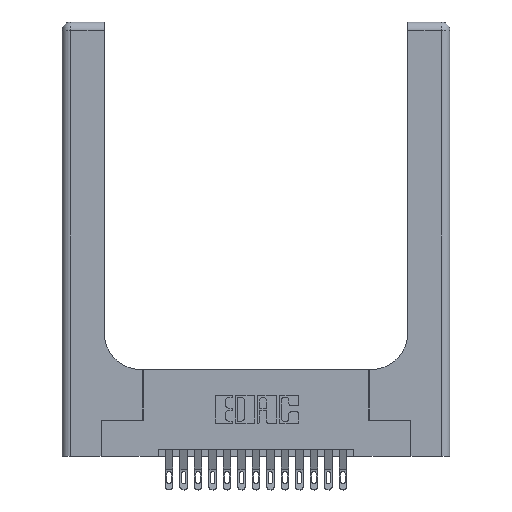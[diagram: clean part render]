
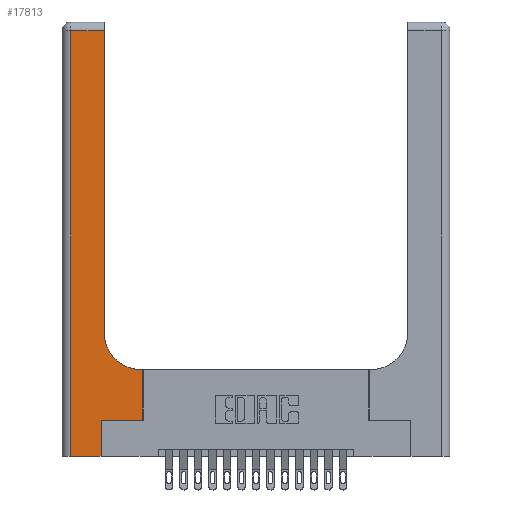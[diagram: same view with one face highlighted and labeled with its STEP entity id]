
A CAD part, top view. The second image highlights one B-rep face of the part: STEP entity #17813.
In plain terms, the highlighted planar face has unit normal (0, 0, 1).
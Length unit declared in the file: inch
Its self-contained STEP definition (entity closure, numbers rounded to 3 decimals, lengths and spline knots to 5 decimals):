
#219 = VERTEX_POINT ( 'NONE', #9522 ) ;
#544 = VERTEX_POINT ( 'NONE', #1784 ) ;
#628 = AXIS2_PLACEMENT_3D ( 'NONE', #1355, #11418, #13408 ) ;
#735 = LINE ( 'NONE', #16271, #17061 ) ;
#807 = DIRECTION ( 'NONE',  ( 1., 0., 0. ) ) ;
#1086 = EDGE_LOOP ( 'NONE', ( #16176, #7851, #3524, #15722, #14013, #7031, #16193, #15386, #12107 ) ) ;
#1355 = CARTESIAN_POINT ( 'NONE',  ( 0., 3., 0.37 ) ) ;
#1466 = LINE ( 'NONE', #12705, #5020 ) ;
#1563 = CARTESIAN_POINT ( 'NONE',  ( 0.06, 2.94, 0.37 ) ) ;
#1784 = CARTESIAN_POINT ( 'NONE',  ( 0.2915, 0.85, 0.37 ) ) ;
#1847 = EDGE_CURVE ( 'NONE', #13641, #544, #18975, .T. ) ;
#1978 = CARTESIAN_POINT ( 'NONE',  ( 0.5585, 0.6, 0.37 ) ) ;
#2128 = CARTESIAN_POINT ( 'NONE',  ( 0.5415, 0.6, 0.37 ) ) ;
#2140 = CARTESIAN_POINT ( 'NONE',  ( 0.269, 0.25, 0.37 ) ) ;
#2630 = VECTOR ( 'NONE', #8800, 39.37008 ) ;
#3524 = ORIENTED_EDGE ( 'NONE', *, *, #8120, .T. ) ;
#3537 = VECTOR ( 'NONE', #17474, 39.37008 ) ;
#4031 = LINE ( 'NONE', #13912, #3537 ) ;
#5020 = VECTOR ( 'NONE', #807, 39.37008 ) ;
#5067 = CARTESIAN_POINT ( 'NONE',  ( 0.2915, 0.6, 0.37 ) ) ;
#5186 = CARTESIAN_POINT ( 'NONE',  ( 0.06, 3., 0.37 ) ) ;
#5453 = AXIS2_PLACEMENT_3D ( 'NONE', #8823, #17914, #10262 ) ;
#6073 = VECTOR ( 'NONE', #14108, 39.37008 ) ;
#7031 = ORIENTED_EDGE ( 'NONE', *, *, #15122, .T. ) ;
#7089 = CARTESIAN_POINT ( 'NONE',  ( 0.269, 0., 0.37 ) ) ;
#7225 = DIRECTION ( 'NONE',  ( 0., 1., 0. ) ) ;
#7851 = ORIENTED_EDGE ( 'NONE', *, *, #9613, .T. ) ;
#8120 = EDGE_CURVE ( 'NONE', #12948, #219, #14992, .T. ) ;
#8372 = LINE ( 'NONE', #5067, #12856 ) ;
#8697 = EDGE_CURVE ( 'NONE', #14667, #13161, #735, .T. ) ;
#8800 = DIRECTION ( 'NONE',  ( -1., 0., 0. ) ) ;
#8823 = CARTESIAN_POINT ( 'NONE',  ( 0.5415, 0.85, 0.37 ) ) ;
#8880 = FACE_OUTER_BOUND ( 'NONE', #1086, .T. ) ;
#8973 = VERTEX_POINT ( 'NONE', #1978 ) ;
#9394 = LINE ( 'NONE', #2140, #6073 ) ;
#9522 = CARTESIAN_POINT ( 'NONE',  ( 0.06, 0., 0.37 ) ) ;
#9544 = DIRECTION ( 'NONE',  ( 0., -1., 0. ) ) ;
#9613 = EDGE_CURVE ( 'NONE', #19587, #12948, #11138, .T. ) ;
#10262 = DIRECTION ( 'NONE',  ( 1., 0., 0. ) ) ;
#10984 = EDGE_CURVE ( 'NONE', #12523, #8973, #4031, .T. ) ;
#11138 = LINE ( 'NONE', #11352, #2630 ) ;
#11298 = CARTESIAN_POINT ( 'NONE',  ( 0.5585, 0.25, 0.37 ) ) ;
#11352 = CARTESIAN_POINT ( 'NONE',  ( 0., 2.94, 0.37 ) ) ;
#11418 = DIRECTION ( 'NONE',  ( 0., 0., -1. ) ) ;
#11547 = CARTESIAN_POINT ( 'NONE',  ( 0.2915, 2.94, 0.37 ) ) ;
#11973 = EDGE_CURVE ( 'NONE', #219, #14667, #1466, .T. ) ;
#12107 = ORIENTED_EDGE ( 'NONE', *, *, #1847, .T. ) ;
#12523 = VERTEX_POINT ( 'NONE', #11298 ) ;
#12705 = CARTESIAN_POINT ( 'NONE',  ( 0., 0., 0.37 ) ) ;
#12726 = CARTESIAN_POINT ( 'NONE',  ( 0.269, 0.25, 0.37 ) ) ;
#12856 = VECTOR ( 'NONE', #12861, 39.37008 ) ;
#12861 = DIRECTION ( 'NONE',  ( -1., 0., 0. ) ) ;
#12931 = EDGE_CURVE ( 'NONE', #544, #19587, #14189, .T. ) ;
#12948 = VERTEX_POINT ( 'NONE', #1563 ) ;
#13161 = VERTEX_POINT ( 'NONE', #12726 ) ;
#13408 = DIRECTION ( 'NONE',  ( -1., 0., 0. ) ) ;
#13641 = VERTEX_POINT ( 'NONE', #2128 ) ;
#13912 = CARTESIAN_POINT ( 'NONE',  ( 0.5585, 0.25, 0.37 ) ) ;
#14013 = ORIENTED_EDGE ( 'NONE', *, *, #8697, .T. ) ;
#14108 = DIRECTION ( 'NONE',  ( 1., 0., 0. ) ) ;
#14189 = LINE ( 'NONE', #17994, #18922 ) ;
#14265 = VECTOR ( 'NONE', #9544, 39.37008 ) ;
#14667 = VERTEX_POINT ( 'NONE', #7089 ) ;
#14866 = PLANE ( 'NONE',  #628 ) ;
#14992 = LINE ( 'NONE', #5186, #14265 ) ;
#15122 = EDGE_CURVE ( 'NONE', #13161, #12523, #9394, .T. ) ;
#15386 = ORIENTED_EDGE ( 'NONE', *, *, #17578, .T. ) ;
#15722 = ORIENTED_EDGE ( 'NONE', *, *, #11973, .T. ) ;
#16176 = ORIENTED_EDGE ( 'NONE', *, *, #12931, .T. ) ;
#16193 = ORIENTED_EDGE ( 'NONE', *, *, #10984, .T. ) ;
#16271 = CARTESIAN_POINT ( 'NONE',  ( 0.269, 0., 0.37 ) ) ;
#16601 = DIRECTION ( 'NONE',  ( 0., 1., 0. ) ) ;
#17061 = VECTOR ( 'NONE', #7225, 39.37008 ) ;
#17474 = DIRECTION ( 'NONE',  ( 0., 1., 0. ) ) ;
#17578 = EDGE_CURVE ( 'NONE', #8973, #13641, #8372, .T. ) ;
#17813 = ADVANCED_FACE ( 'NONE', ( #8880 ), #14866, .F. ) ;
#17914 = DIRECTION ( 'NONE',  ( 0., 0., -1. ) ) ;
#17994 = CARTESIAN_POINT ( 'NONE',  ( 0.2915, 3., 0.37 ) ) ;
#18922 = VECTOR ( 'NONE', #16601, 39.37008 ) ;
#18975 = CIRCLE ( 'NONE', #5453, 0.25 ) ;
#19587 = VERTEX_POINT ( 'NONE', #11547 ) ;
